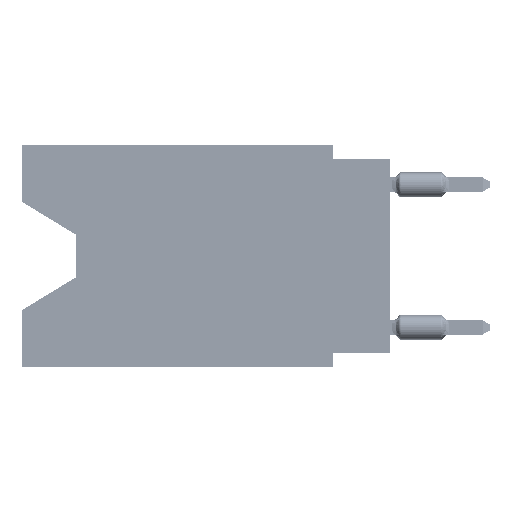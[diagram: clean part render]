
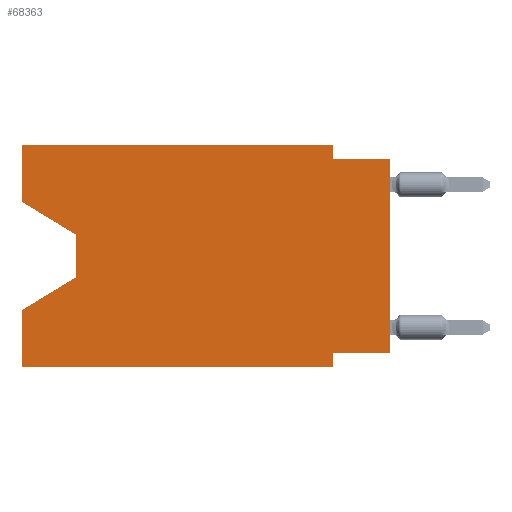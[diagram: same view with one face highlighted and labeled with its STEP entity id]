
A CAD part, left-side view. The second image highlights one B-rep face of the part: STEP entity #68363.
In plain terms, the highlighted planar face has unit normal (-1, 0, 0).
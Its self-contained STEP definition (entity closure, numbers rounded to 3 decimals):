
#2446 = LINE ( 'NONE', #2839, #21188 ) ;
#2839 = CARTESIAN_POINT ( 'NONE',  ( 0., 0., -9.271 ) ) ;
#3028 = LINE ( 'NONE', #46471, #50390 ) ;
#4384 = ORIENTED_EDGE ( 'NONE', *, *, #59820, .T. ) ;
#4601 = LINE ( 'NONE', #48448, #77341 ) ;
#5051 = DIRECTION ( 'NONE',  ( 0., 0., 1. ) ) ;
#7724 = EDGE_CURVE ( 'NONE', #52922, #17866, #17170, .T. ) ;
#8948 = VECTOR ( 'NONE', #30629, 1000. ) ;
#11606 = VERTEX_POINT ( 'NONE', #20276 ) ;
#11748 = CARTESIAN_POINT ( 'NONE',  ( 0., 16.383, -9.906 ) ) ;
#11822 = CARTESIAN_POINT ( 'NONE',  ( 0., 13.97, -5.893 ) ) ;
#14624 = DIRECTION ( 'NONE',  ( 0., -1., 0. ) ) ;
#17170 = LINE ( 'NONE', #59816, #37917 ) ;
#17187 = DIRECTION ( 'NONE',  ( 0., 0., 1. ) ) ;
#17564 = VERTEX_POINT ( 'NONE', #56786 ) ;
#17730 = CARTESIAN_POINT ( 'NONE',  ( 0., 2.54, -0.635 ) ) ;
#17866 = VERTEX_POINT ( 'NONE', #17730 ) ;
#18286 = ORIENTED_EDGE ( 'NONE', *, *, #35272, .F. ) ;
#18838 = LINE ( 'NONE', #26154, #35271 ) ;
#19760 = EDGE_CURVE ( 'NONE', #35653, #35134, #18838, .T. ) ;
#20276 = CARTESIAN_POINT ( 'NONE',  ( 0., 0., -0.635 ) ) ;
#21188 = VECTOR ( 'NONE', #52372, 1000. ) ;
#22580 = DIRECTION ( 'NONE',  ( 0., 0., 1. ) ) ;
#22664 = CARTESIAN_POINT ( 'NONE',  ( 0., 2.54, -9.906 ) ) ;
#23976 = VECTOR ( 'NONE', #5051, 1000. ) ;
#24019 = EDGE_LOOP ( 'NONE', ( #72884, #62484, #37625, #36072, #41354, #59573, #18286, #4384, #68792, #57092, #51156, #55814 ) ) ;
#26154 = CARTESIAN_POINT ( 'NONE',  ( 0., 13.97, -4.013 ) ) ;
#27327 = VERTEX_POINT ( 'NONE', #34007 ) ;
#28680 = LINE ( 'NONE', #40436, #58216 ) ;
#30187 = DIRECTION ( 'NONE',  ( 0., 0., -1. ) ) ;
#30629 = DIRECTION ( 'NONE',  ( 0., 0., -1. ) ) ;
#31079 = EDGE_CURVE ( 'NONE', #17564, #66189, #31427, .T. ) ;
#31427 = LINE ( 'NONE', #50521, #8948 ) ;
#31709 = CARTESIAN_POINT ( 'NONE',  ( 0., 0., -0.635 ) ) ;
#31826 = DIRECTION ( 'NONE',  ( 0., 0., -1. ) ) ;
#34007 = CARTESIAN_POINT ( 'NONE',  ( 0., 16.383, 0. ) ) ;
#35134 = VERTEX_POINT ( 'NONE', #11822 ) ;
#35271 = VECTOR ( 'NONE', #31826, 1000. ) ;
#35272 = EDGE_CURVE ( 'NONE', #49130, #17564, #2446, .T. ) ;
#35653 = VERTEX_POINT ( 'NONE', #49077 ) ;
#36072 = ORIENTED_EDGE ( 'NONE', *, *, #55135, .F. ) ;
#37625 = ORIENTED_EDGE ( 'NONE', *, *, #47617, .T. ) ;
#37917 = VECTOR ( 'NONE', #60609, 1000. ) ;
#38142 = EDGE_CURVE ( 'NONE', #50337, #27327, #40781, .T. ) ;
#39053 = CARTESIAN_POINT ( 'NONE',  ( 0., 16.383, 0. ) ) ;
#40436 = CARTESIAN_POINT ( 'NONE',  ( 0., 0., 0. ) ) ;
#40746 = CARTESIAN_POINT ( 'NONE',  ( 0., 16.383, -2.546 ) ) ;
#40781 = LINE ( 'NONE', #78953, #23976 ) ;
#41354 = ORIENTED_EDGE ( 'NONE', *, *, #72254, .T. ) ;
#46028 = CARTESIAN_POINT ( 'NONE',  ( 0., 16.383, -9.906 ) ) ;
#46471 = CARTESIAN_POINT ( 'NONE',  ( 0., 13.97, -5.893 ) ) ;
#46856 = CARTESIAN_POINT ( 'NONE',  ( 0., 16.383, -2.546 ) ) ;
#47617 = EDGE_CURVE ( 'NONE', #35134, #75896, #3028, .T. ) ;
#48004 = VECTOR ( 'NONE', #59439, 1000. ) ;
#48062 = PLANE ( 'NONE',  #75956 ) ;
#48448 = CARTESIAN_POINT ( 'NONE',  ( 0., 16.383, 0. ) ) ;
#48849 = EDGE_CURVE ( 'NONE', #27327, #52922, #64207, .T. ) ;
#49044 = VECTOR ( 'NONE', #63433, 1000. ) ;
#49077 = CARTESIAN_POINT ( 'NONE',  ( 0., 13.97, -4.013 ) ) ;
#49130 = VERTEX_POINT ( 'NONE', #68208 ) ;
#49365 = CARTESIAN_POINT ( 'NONE',  ( 0., 16.383, -7.36 ) ) ;
#49892 = DIRECTION ( 'NONE',  ( 0., -1., 0. ) ) ;
#50337 = VERTEX_POINT ( 'NONE', #46856 ) ;
#50390 = VECTOR ( 'NONE', #71225, 1000. ) ;
#50521 = CARTESIAN_POINT ( 'NONE',  ( 0., 2.54, -9.906 ) ) ;
#50793 = LINE ( 'NONE', #31709, #68194 ) ;
#51156 = ORIENTED_EDGE ( 'NONE', *, *, #48849, .F. ) ;
#52372 = DIRECTION ( 'NONE',  ( 0., 1., 0. ) ) ;
#52922 = VERTEX_POINT ( 'NONE', #57623 ) ;
#55135 = EDGE_CURVE ( 'NONE', #66400, #75896, #4601, .T. ) ;
#55814 = ORIENTED_EDGE ( 'NONE', *, *, #38142, .F. ) ;
#56786 = CARTESIAN_POINT ( 'NONE',  ( 0., 2.54, -9.271 ) ) ;
#57092 = ORIENTED_EDGE ( 'NONE', *, *, #7724, .F. ) ;
#57623 = CARTESIAN_POINT ( 'NONE',  ( 0., 2.54, 0. ) ) ;
#58216 = VECTOR ( 'NONE', #22580, 1000. ) ;
#59439 = DIRECTION ( 'NONE',  ( 0., -0.855, -0.519 ) ) ;
#59573 = ORIENTED_EDGE ( 'NONE', *, *, #31079, .F. ) ;
#59816 = CARTESIAN_POINT ( 'NONE',  ( 0., 2.54, 0. ) ) ;
#59820 = EDGE_CURVE ( 'NONE', #49130, #11606, #28680, .T. ) ;
#59840 = LINE ( 'NONE', #40746, #48004 ) ;
#60240 = FACE_OUTER_BOUND ( 'NONE', #24019, .T. ) ;
#60609 = DIRECTION ( 'NONE',  ( 0., 0., -1. ) ) ;
#61041 = CARTESIAN_POINT ( 'NONE',  ( 0., 16.383, 0. ) ) ;
#61531 = EDGE_CURVE ( 'NONE', #50337, #35653, #59840, .T. ) ;
#62484 = ORIENTED_EDGE ( 'NONE', *, *, #19760, .T. ) ;
#63433 = DIRECTION ( 'NONE',  ( 0., -1., 0. ) ) ;
#64207 = LINE ( 'NONE', #39053, #49044 ) ;
#66189 = VERTEX_POINT ( 'NONE', #22664 ) ;
#66400 = VERTEX_POINT ( 'NONE', #46028 ) ;
#66472 = VECTOR ( 'NONE', #49892, 1000. ) ;
#68194 = VECTOR ( 'NONE', #14624, 1000. ) ;
#68208 = CARTESIAN_POINT ( 'NONE',  ( 0., 0., -9.271 ) ) ;
#68363 = ADVANCED_FACE ( 'NONE', ( #60240 ), #48062, .F. ) ;
#68561 = LINE ( 'NONE', #11748, #66472 ) ;
#68792 = ORIENTED_EDGE ( 'NONE', *, *, #77977, .F. ) ;
#71225 = DIRECTION ( 'NONE',  ( 0., 0.855, -0.519 ) ) ;
#72254 = EDGE_CURVE ( 'NONE', #66400, #66189, #68561, .T. ) ;
#72884 = ORIENTED_EDGE ( 'NONE', *, *, #61531, .T. ) ;
#75896 = VERTEX_POINT ( 'NONE', #49365 ) ;
#75956 = AXIS2_PLACEMENT_3D ( 'NONE', #61041, #78926, #30187 ) ;
#77341 = VECTOR ( 'NONE', #17187, 1000. ) ;
#77977 = EDGE_CURVE ( 'NONE', #17866, #11606, #50793, .T. ) ;
#78926 = DIRECTION ( 'NONE',  ( 1., 0., 0. ) ) ;
#78953 = CARTESIAN_POINT ( 'NONE',  ( 0., 16.383, 0. ) ) ;
